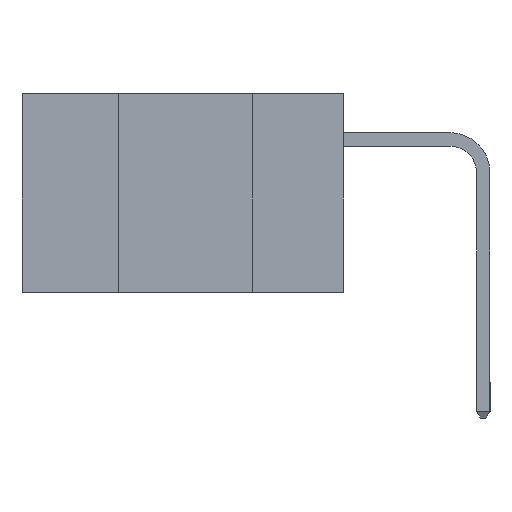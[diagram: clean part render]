
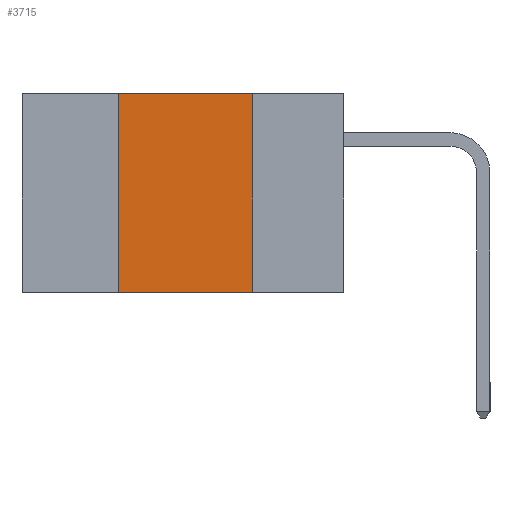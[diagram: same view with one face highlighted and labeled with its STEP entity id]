
A CAD part, left-side view. The second image highlights one B-rep face of the part: STEP entity #3715.
In plain terms, the highlighted planar face has unit normal (-1, 0, 0).
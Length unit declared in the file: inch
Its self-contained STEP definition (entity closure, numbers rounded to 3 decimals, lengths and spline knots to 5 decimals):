
#443 = FACE_OUTER_BOUND ( 'NONE', #10267, .T. ) ;
#1919 = DIRECTION ( 'NONE',  ( 0., -1., 0. ) ) ;
#2065 = VECTOR ( 'NONE', #13960, 39.37008 ) ;
#2396 = CARTESIAN_POINT ( 'NONE',  ( 0., 0.42, -0.37 ) ) ;
#2648 = DIRECTION ( 'NONE',  ( 1., 0., 0. ) ) ;
#3309 = CARTESIAN_POINT ( 'NONE',  ( 0., 0.42, 0. ) ) ;
#3713 = ORIENTED_EDGE ( 'NONE', *, *, #4633, .F. ) ;
#3715 = ADVANCED_FACE ( 'NONE', ( #443 ), #9101, .F. ) ;
#4052 = CARTESIAN_POINT ( 'NONE',  ( 0., 0.42, -0.37 ) ) ;
#4633 = EDGE_CURVE ( 'NONE', #13619, #10919, #8079, .T. ) ;
#5086 = ORIENTED_EDGE ( 'NONE', *, *, #6711, .F. ) ;
#5106 = LINE ( 'NONE', #7368, #5537 ) ;
#5118 = CARTESIAN_POINT ( 'NONE',  ( 0., 0.17, 0. ) ) ;
#5537 = VECTOR ( 'NONE', #1919, 39.37008 ) ;
#5714 = ORIENTED_EDGE ( 'NONE', *, *, #5750, .F. ) ;
#5750 = EDGE_CURVE ( 'NONE', #13440, #13619, #11295, .T. ) ;
#5984 = CARTESIAN_POINT ( 'NONE',  ( 0., 0.17, -0.37 ) ) ;
#6711 = EDGE_CURVE ( 'NONE', #10415, #13440, #12888, .T. ) ;
#6884 = DIRECTION ( 'NONE',  ( 0., -1., 0. ) ) ;
#6973 = DIRECTION ( 'NONE',  ( 0., 0., -1. ) ) ;
#7012 = CARTESIAN_POINT ( 'NONE',  ( 0., 0.17, -0.37 ) ) ;
#7368 = CARTESIAN_POINT ( 'NONE',  ( 0., 0.6, -0.37 ) ) ;
#7785 = VECTOR ( 'NONE', #13591, 39.37008 ) ;
#8028 = CARTESIAN_POINT ( 'NONE',  ( 0., 0.6, 0. ) ) ;
#8079 = LINE ( 'NONE', #7012, #7785 ) ;
#8873 = CARTESIAN_POINT ( 'NONE',  ( 0., 0.6, 0. ) ) ;
#9101 = PLANE ( 'NONE',  #13243 ) ;
#9509 = EDGE_CURVE ( 'NONE', #10415, #10919, #5106, .T. ) ;
#10267 = EDGE_LOOP ( 'NONE', ( #3713, #5714, #5086, #11211 ) ) ;
#10415 = VERTEX_POINT ( 'NONE', #2396 ) ;
#10919 = VERTEX_POINT ( 'NONE', #5984 ) ;
#11211 = ORIENTED_EDGE ( 'NONE', *, *, #9509, .T. ) ;
#11295 = LINE ( 'NONE', #8873, #11859 ) ;
#11859 = VECTOR ( 'NONE', #6884, 39.37008 ) ;
#12888 = LINE ( 'NONE', #4052, #2065 ) ;
#13243 = AXIS2_PLACEMENT_3D ( 'NONE', #8028, #2648, #6973 ) ;
#13440 = VERTEX_POINT ( 'NONE', #3309 ) ;
#13591 = DIRECTION ( 'NONE',  ( 0., 0., -1. ) ) ;
#13619 = VERTEX_POINT ( 'NONE', #5118 ) ;
#13960 = DIRECTION ( 'NONE',  ( 0., 0., 1. ) ) ;
